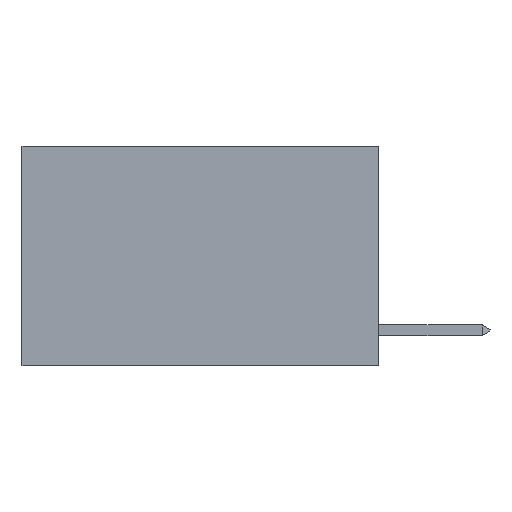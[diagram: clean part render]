
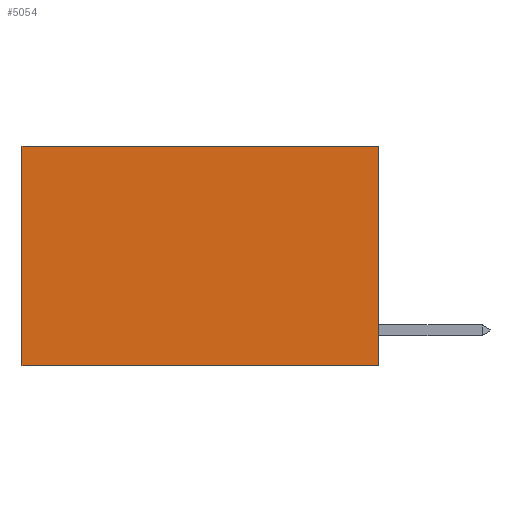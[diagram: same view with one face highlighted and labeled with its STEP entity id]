
A CAD part, left-side view. The second image highlights one B-rep face of the part: STEP entity #5054.
In plain terms, the highlighted planar face has unit normal (-1, 0, 0).
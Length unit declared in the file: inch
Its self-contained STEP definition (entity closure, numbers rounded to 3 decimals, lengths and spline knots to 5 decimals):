
#117 = VERTEX_POINT ( 'NONE', #5230 ) ;
#236 = EDGE_CURVE ( 'NONE', #117, #7981, #6467, .T. ) ;
#534 = EDGE_CURVE ( 'NONE', #11063, #7981, #10848, .T. ) ;
#692 = PLANE ( 'NONE',  #7031 ) ;
#1103 = EDGE_LOOP ( 'NONE', ( #1942, #2309, #1969, #4797 ) ) ;
#1142 = DIRECTION ( 'NONE',  ( 0., 0., -1. ) ) ;
#1292 = VECTOR ( 'NONE', #2932, 39.37008 ) ;
#1376 = EDGE_CURVE ( 'NONE', #5568, #117, #10046, .T. ) ;
#1942 = ORIENTED_EDGE ( 'NONE', *, *, #236, .T. ) ;
#1969 = ORIENTED_EDGE ( 'NONE', *, *, #6085, .F. ) ;
#2210 = LINE ( 'NONE', #6752, #4163 ) ;
#2309 = ORIENTED_EDGE ( 'NONE', *, *, #534, .F. ) ;
#2478 = CARTESIAN_POINT ( 'NONE',  ( 0.2625, 0., -0.37 ) ) ;
#2719 = CARTESIAN_POINT ( 'NONE',  ( 0.2625, 0., 0. ) ) ;
#2932 = DIRECTION ( 'NONE',  ( 0., 0., -1. ) ) ;
#3140 = VECTOR ( 'NONE', #4200, 39.37008 ) ;
#4163 = VECTOR ( 'NONE', #1142, 39.37008 ) ;
#4200 = DIRECTION ( 'NONE',  ( 0., 1., 0. ) ) ;
#4603 = CARTESIAN_POINT ( 'NONE',  ( 0.2625, 0.6, 0. ) ) ;
#4797 = ORIENTED_EDGE ( 'NONE', *, *, #1376, .T. ) ;
#5054 = ADVANCED_FACE ( 'NONE', ( #9232 ), #692, .F. ) ;
#5230 = CARTESIAN_POINT ( 'NONE',  ( 0.2625, 0.6, 0. ) ) ;
#5568 = VERTEX_POINT ( 'NONE', #7473 ) ;
#6046 = CARTESIAN_POINT ( 'NONE',  ( 0.2625, 0.6, -0.37 ) ) ;
#6085 = EDGE_CURVE ( 'NONE', #5568, #11063, #2210, .T. ) ;
#6467 = LINE ( 'NONE', #4603, #1292 ) ;
#6752 = CARTESIAN_POINT ( 'NONE',  ( 0.2625, 0., 0. ) ) ;
#7031 = AXIS2_PLACEMENT_3D ( 'NONE', #2719, #11965, #8292 ) ;
#7473 = CARTESIAN_POINT ( 'NONE',  ( 0.2625, 0., 0. ) ) ;
#7981 = VERTEX_POINT ( 'NONE', #6046 ) ;
#8076 = CARTESIAN_POINT ( 'NONE',  ( 0.2625, 0., 0. ) ) ;
#8292 = DIRECTION ( 'NONE',  ( 0., 0., -1. ) ) ;
#9232 = FACE_OUTER_BOUND ( 'NONE', #1103, .T. ) ;
#10046 = LINE ( 'NONE', #8076, #11688 ) ;
#10848 = LINE ( 'NONE', #2478, #3140 ) ;
#11040 = DIRECTION ( 'NONE',  ( 0., 1., 0. ) ) ;
#11063 = VERTEX_POINT ( 'NONE', #11793 ) ;
#11688 = VECTOR ( 'NONE', #11040, 39.37008 ) ;
#11793 = CARTESIAN_POINT ( 'NONE',  ( 0.2625, 0., -0.37 ) ) ;
#11965 = DIRECTION ( 'NONE',  ( 1., 0., 0. ) ) ;
